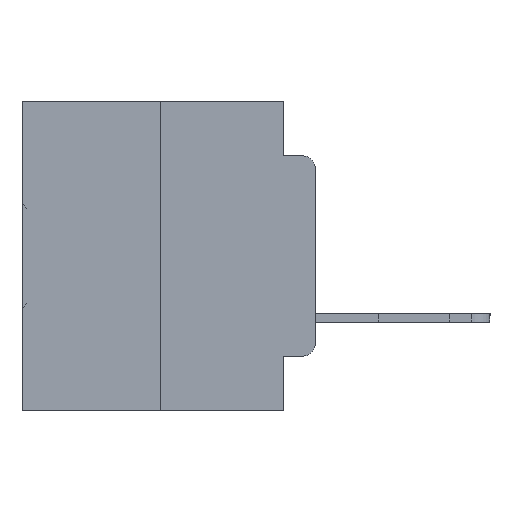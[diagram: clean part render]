
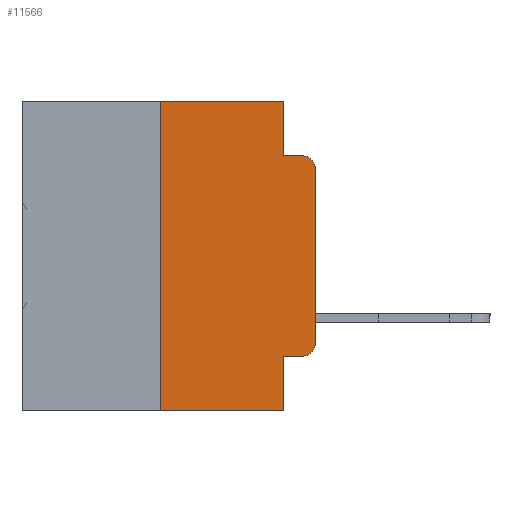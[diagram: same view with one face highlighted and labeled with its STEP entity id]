
A CAD part, left-side view. The second image highlights one B-rep face of the part: STEP entity #11566.
In plain terms, the highlighted planar face has unit normal (-1, 0, 0).
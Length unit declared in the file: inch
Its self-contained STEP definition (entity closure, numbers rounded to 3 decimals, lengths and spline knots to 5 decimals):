
#77 = CARTESIAN_POINT ( 'NONE',  ( 0., 0.473, 0. ) ) ;
#436 = ORIENTED_EDGE ( 'NONE', *, *, #34512, .T. ) ;
#628 = VERTEX_POINT ( 'NONE', #7288 ) ;
#1915 = VERTEX_POINT ( 'NONE', #4123 ) ;
#2015 = VERTEX_POINT ( 'NONE', #23432 ) ;
#2160 = DIRECTION ( 'NONE',  ( 1., 0., 0. ) ) ;
#2277 = CARTESIAN_POINT ( 'NONE',  ( 0., 0.051, 0. ) ) ;
#2829 = CARTESIAN_POINT ( 'NONE',  ( 0., 0.02, -0.0885 ) ) ;
#2880 = DIRECTION ( 'NONE',  ( 0., -1., 0. ) ) ;
#3069 = CARTESIAN_POINT ( 'NONE',  ( 0., 0.051, -0.0885 ) ) ;
#4123 = CARTESIAN_POINT ( 'NONE',  ( 0., 0., -0.3915 ) ) ;
#4316 = ORIENTED_EDGE ( 'NONE', *, *, #16210, .F. ) ;
#4717 = VECTOR ( 'NONE', #2880, 39.37008 ) ;
#5301 = EDGE_CURVE ( 'NONE', #6082, #8836, #7807, .T. ) ;
#5359 = CARTESIAN_POINT ( 'NONE',  ( 0., 0., 0. ) ) ;
#5578 = FACE_OUTER_BOUND ( 'NONE', #25920, .T. ) ;
#5854 = DIRECTION ( 'NONE',  ( 0., -1., 0. ) ) ;
#6011 = VERTEX_POINT ( 'NONE', #2829 ) ;
#6082 = VERTEX_POINT ( 'NONE', #29962 ) ;
#7288 = CARTESIAN_POINT ( 'NONE',  ( 0., 0., -0.1085 ) ) ;
#7581 = VERTEX_POINT ( 'NONE', #25877 ) ;
#7599 = PLANE ( 'NONE',  #25327 ) ;
#7807 = LINE ( 'NONE', #2277, #21310 ) ;
#8108 = DIRECTION ( 'NONE',  ( 0., 0., 1. ) ) ;
#8135 = LINE ( 'NONE', #15836, #14491 ) ;
#8651 = ORIENTED_EDGE ( 'NONE', *, *, #9253, .T. ) ;
#8836 = VERTEX_POINT ( 'NONE', #32185 ) ;
#8858 = AXIS2_PLACEMENT_3D ( 'NONE', #14774, #33207, #17508 ) ;
#9253 = EDGE_CURVE ( 'NONE', #20523, #8836, #27078, .T. ) ;
#9494 = LINE ( 'NONE', #12160, #14979 ) ;
#9788 = VERTEX_POINT ( 'NONE', #26077 ) ;
#10808 = EDGE_CURVE ( 'NONE', #20523, #2015, #9494, .T. ) ;
#11566 = ADVANCED_FACE ( 'NONE', ( #5578 ), #7599, .F. ) ;
#12041 = DIRECTION ( 'NONE',  ( 0., 0., 1. ) ) ;
#12160 = CARTESIAN_POINT ( 'NONE',  ( 0., 0.25, 0. ) ) ;
#12546 = DIRECTION ( 'NONE',  ( -1., 0., 0. ) ) ;
#12550 = ORIENTED_EDGE ( 'NONE', *, *, #32713, .T. ) ;
#13269 = ORIENTED_EDGE ( 'NONE', *, *, #10808, .F. ) ;
#13913 = ORIENTED_EDGE ( 'NONE', *, *, #29026, .T. ) ;
#14191 = ORIENTED_EDGE ( 'NONE', *, *, #5301, .F. ) ;
#14491 = VECTOR ( 'NONE', #29736, 39.37008 ) ;
#14774 = CARTESIAN_POINT ( 'NONE',  ( 0., 0.02, -0.3915 ) ) ;
#14979 = VECTOR ( 'NONE', #12041, 39.37008 ) ;
#15836 = CARTESIAN_POINT ( 'NONE',  ( 0., 0.051, 0. ) ) ;
#15842 = CARTESIAN_POINT ( 'NONE',  ( 0., 0.473, -0.5 ) ) ;
#15965 = DIRECTION ( 'NONE',  ( 0., -1., 0. ) ) ;
#16210 = EDGE_CURVE ( 'NONE', #28877, #7581, #8135, .T. ) ;
#17508 = DIRECTION ( 'NONE',  ( 0., 0., -1. ) ) ;
#18047 = EDGE_CURVE ( 'NONE', #7581, #6011, #20685, .T. ) ;
#18528 = CARTESIAN_POINT ( 'NONE',  ( 0., 0.473, 0. ) ) ;
#18811 = ORIENTED_EDGE ( 'NONE', *, *, #34574, .F. ) ;
#18906 = CIRCLE ( 'NONE', #28495, 0.02 ) ;
#18971 = CIRCLE ( 'NONE', #8858, 0.02 ) ;
#19028 = ORIENTED_EDGE ( 'NONE', *, *, #25524, .T. ) ;
#19188 = LINE ( 'NONE', #77, #4717 ) ;
#20169 = VECTOR ( 'NONE', #15965, 39.37008 ) ;
#20523 = VERTEX_POINT ( 'NONE', #33516 ) ;
#20685 = LINE ( 'NONE', #3069, #32900 ) ;
#21183 = DIRECTION ( 'NONE',  ( 0., 0., -1. ) ) ;
#21310 = VECTOR ( 'NONE', #23863, 39.37008 ) ;
#21652 = VECTOR ( 'NONE', #29348, 39.37008 ) ;
#22437 = LINE ( 'NONE', #26726, #21652 ) ;
#23432 = CARTESIAN_POINT ( 'NONE',  ( 0., 0.25, 0. ) ) ;
#23863 = DIRECTION ( 'NONE',  ( 0., 0., -1. ) ) ;
#25327 = AXIS2_PLACEMENT_3D ( 'NONE', #18528, #2160, #21183 ) ;
#25524 = EDGE_CURVE ( 'NONE', #628, #6011, #18906, .T. ) ;
#25877 = CARTESIAN_POINT ( 'NONE',  ( 0., 0.051, -0.0885 ) ) ;
#25920 = EDGE_LOOP ( 'NONE', ( #13913, #19028, #33912, #4316, #18811, #13269, #8651, #14191, #436, #12550 ) ) ;
#26077 = CARTESIAN_POINT ( 'NONE',  ( 0., 0.02, -0.4115 ) ) ;
#26079 = CARTESIAN_POINT ( 'NONE',  ( 0., 0.051, 0. ) ) ;
#26726 = CARTESIAN_POINT ( 'NONE',  ( 0., 0.051, -0.4115 ) ) ;
#27078 = LINE ( 'NONE', #15842, #20169 ) ;
#28415 = CARTESIAN_POINT ( 'NONE',  ( 0., 0.02, -0.1085 ) ) ;
#28495 = AXIS2_PLACEMENT_3D ( 'NONE', #28415, #12546, #31029 ) ;
#28556 = LINE ( 'NONE', #5359, #33894 ) ;
#28877 = VERTEX_POINT ( 'NONE', #26079 ) ;
#29026 = EDGE_CURVE ( 'NONE', #1915, #628, #28556, .T. ) ;
#29348 = DIRECTION ( 'NONE',  ( 0., -1., 0. ) ) ;
#29736 = DIRECTION ( 'NONE',  ( 0., 0., -1. ) ) ;
#29962 = CARTESIAN_POINT ( 'NONE',  ( 0., 0.051, -0.4115 ) ) ;
#31029 = DIRECTION ( 'NONE',  ( 0., 0., -1. ) ) ;
#32185 = CARTESIAN_POINT ( 'NONE',  ( 0., 0.051, -0.5 ) ) ;
#32713 = EDGE_CURVE ( 'NONE', #9788, #1915, #18971, .T. ) ;
#32900 = VECTOR ( 'NONE', #5854, 39.37008 ) ;
#33207 = DIRECTION ( 'NONE',  ( -1., 0., 0. ) ) ;
#33516 = CARTESIAN_POINT ( 'NONE',  ( 0., 0.25, -0.5 ) ) ;
#33894 = VECTOR ( 'NONE', #8108, 39.37008 ) ;
#33912 = ORIENTED_EDGE ( 'NONE', *, *, #18047, .F. ) ;
#34512 = EDGE_CURVE ( 'NONE', #6082, #9788, #22437, .T. ) ;
#34574 = EDGE_CURVE ( 'NONE', #2015, #28877, #19188, .T. ) ;
